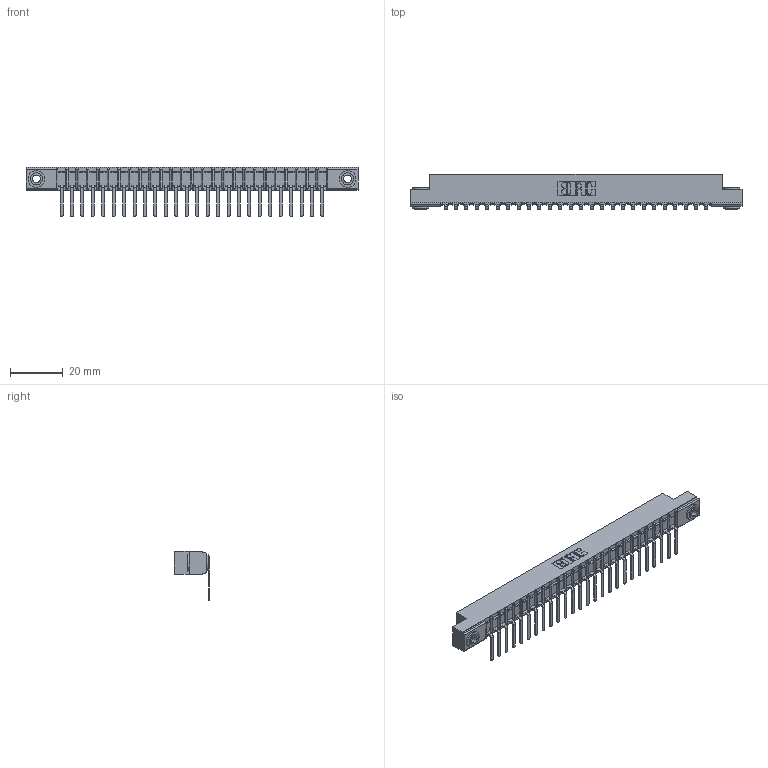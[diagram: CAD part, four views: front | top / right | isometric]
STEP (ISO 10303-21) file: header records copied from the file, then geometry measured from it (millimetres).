
FILE_DESCRIPTION (( 'STEP AP203' ), '1' );
FILE_NAME ('357-026-457-103.STEP', '2020-10-01T17:57:32', ( '' ), ( '' ), 'SwSTEP 2.0', 'SolidWorks 2020', '' );
FILE_SCHEMA (( 'CONFIG_CONTROL_DESIGN' ));
Length unit declared in the file: inch
Products named in the file (4): 307 Part_.156 Dia Mounting Holes; 307-290-002_557; 345-250-002_345-250-002-102; 357-026-457-103
Assembly tree (29 placements, depth 2):
  357-026-457-103
    307 Part_.156 Dia Mounting Holes
    307-290-002_557  x26
    345-250-002_345-250-002-102  x2
Bounding box: 126.03 x 13.36 x 18.67 mm (x, y, z)
Volume: 8394.1 mm3; surface area: 16162.6 mm2
Topology: 29 solids, 29 shells, 2225 faces, 6779 edges, 4442 vertices
Faces by surface type: plane 1316, cylinder 847, sphere 54, cone 8
Entity records: 26181 total; most frequent: CARTESIAN_POINT 4393, ORIENTED_EDGE 4374, DIRECTION 4291, EDGE_CURVE 2187, LINE 1659, VECTOR 1659, VERTEX_POINT 1418, AXIS2_PLACEMENT_3D 1316
